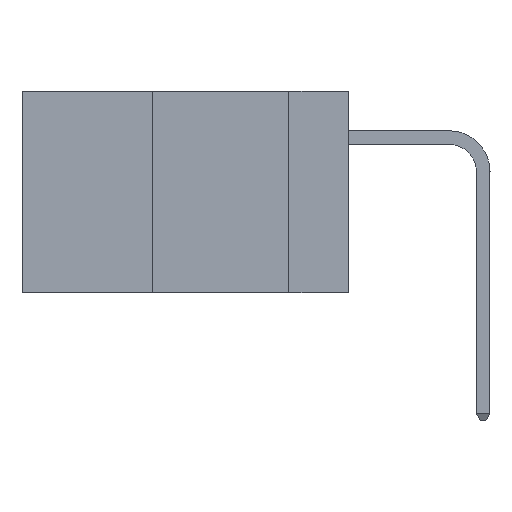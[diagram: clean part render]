
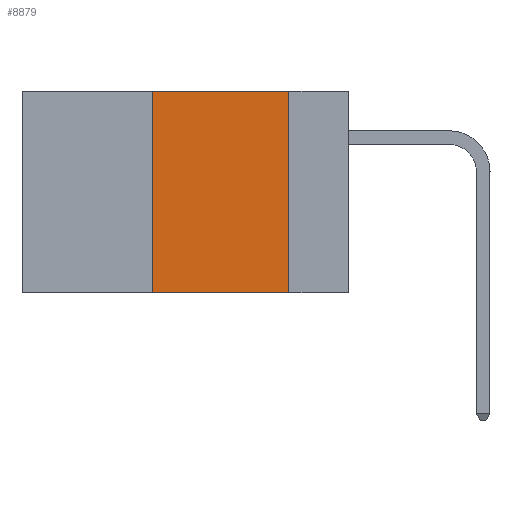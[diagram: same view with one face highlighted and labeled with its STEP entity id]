
A CAD part, left-side view. The second image highlights one B-rep face of the part: STEP entity #8879.
In plain terms, the highlighted planar face has unit normal (-1, 0, 0).
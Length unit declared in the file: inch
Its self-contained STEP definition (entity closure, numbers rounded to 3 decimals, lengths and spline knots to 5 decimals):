
#827 = CARTESIAN_POINT ( 'NONE',  ( 0., 0.6, 0. ) ) ;
#879 = CARTESIAN_POINT ( 'NONE',  ( 0., 0.11, -0.37 ) ) ;
#1307 = CARTESIAN_POINT ( 'NONE',  ( 0., 0.36, 0. ) ) ;
#1378 = CARTESIAN_POINT ( 'NONE',  ( 0., 0.6, 0. ) ) ;
#1547 = ORIENTED_EDGE ( 'NONE', *, *, #6772, .F. ) ;
#2168 = FACE_OUTER_BOUND ( 'NONE', #8053, .T. ) ;
#2209 = LINE ( 'NONE', #2283, #11983 ) ;
#2225 = VECTOR ( 'NONE', #11735, 39.37008 ) ;
#2226 = VERTEX_POINT ( 'NONE', #6137 ) ;
#2283 = CARTESIAN_POINT ( 'NONE',  ( 0., 0.36, 0. ) ) ;
#2373 = VERTEX_POINT ( 'NONE', #1307 ) ;
#2882 = AXIS2_PLACEMENT_3D ( 'NONE', #1378, #5417, #8205 ) ;
#3140 = DIRECTION ( 'NONE',  ( 0., 0., 1. ) ) ;
#3864 = ORIENTED_EDGE ( 'NONE', *, *, #11953, .T. ) ;
#4033 = LINE ( 'NONE', #5952, #5611 ) ;
#4764 = LINE ( 'NONE', #9852, #9814 ) ;
#5417 = DIRECTION ( 'NONE',  ( 1., 0., 0. ) ) ;
#5593 = VERTEX_POINT ( 'NONE', #879 ) ;
#5611 = VECTOR ( 'NONE', #8135, 39.37008 ) ;
#5744 = DIRECTION ( 'NONE',  ( 0., -1., 0. ) ) ;
#5846 = LINE ( 'NONE', #827, #2225 ) ;
#5952 = CARTESIAN_POINT ( 'NONE',  ( 0., 0.11, 0. ) ) ;
#6137 = CARTESIAN_POINT ( 'NONE',  ( 0., 0.11, 0. ) ) ;
#6706 = EDGE_CURVE ( 'NONE', #2226, #5593, #4033, .T. ) ;
#6772 = EDGE_CURVE ( 'NONE', #2373, #2226, #5846, .T. ) ;
#6831 = ORIENTED_EDGE ( 'NONE', *, *, #6706, .F. ) ;
#7806 = CARTESIAN_POINT ( 'NONE',  ( 0., 0.36, -0.37 ) ) ;
#8053 = EDGE_LOOP ( 'NONE', ( #6831, #1547, #10265, #3864 ) ) ;
#8135 = DIRECTION ( 'NONE',  ( 0., 0., -1. ) ) ;
#8205 = DIRECTION ( 'NONE',  ( 0., 0., -1. ) ) ;
#8879 = ADVANCED_FACE ( 'NONE', ( #2168 ), #11236, .F. ) ;
#9613 = EDGE_CURVE ( 'NONE', #10186, #2373, #2209, .T. ) ;
#9814 = VECTOR ( 'NONE', #5744, 39.37008 ) ;
#9852 = CARTESIAN_POINT ( 'NONE',  ( 0., 0.6, -0.37 ) ) ;
#10186 = VERTEX_POINT ( 'NONE', #7806 ) ;
#10265 = ORIENTED_EDGE ( 'NONE', *, *, #9613, .F. ) ;
#11236 = PLANE ( 'NONE',  #2882 ) ;
#11735 = DIRECTION ( 'NONE',  ( 0., -1., 0. ) ) ;
#11953 = EDGE_CURVE ( 'NONE', #10186, #5593, #4764, .T. ) ;
#11983 = VECTOR ( 'NONE', #3140, 39.37008 ) ;
